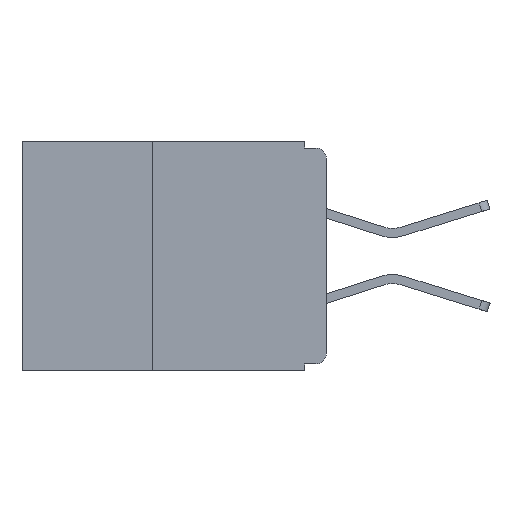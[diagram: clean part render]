
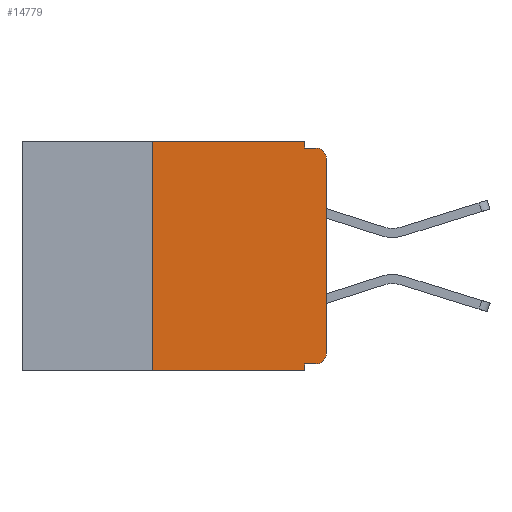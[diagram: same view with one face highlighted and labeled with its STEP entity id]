
A CAD part, left-side view. The second image highlights one B-rep face of the part: STEP entity #14779.
In plain terms, the highlighted planar face has unit normal (-1, 0, 0).
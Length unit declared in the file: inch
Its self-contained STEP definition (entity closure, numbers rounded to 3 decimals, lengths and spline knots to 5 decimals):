
#17 = CARTESIAN_POINT ( 'NONE',  ( 0., 0., -0.32 ) ) ;
#186 = EDGE_CURVE ( 'NONE', #18163, #14115, #7500, .T. ) ;
#317 = CARTESIAN_POINT ( 'NONE',  ( 0., 0.031, -0.01 ) ) ;
#379 = VECTOR ( 'NONE', #11019, 39.37008 ) ;
#574 = LINE ( 'NONE', #5020, #12453 ) ;
#771 = EDGE_CURVE ( 'NONE', #13128, #15462, #13451, .T. ) ;
#1039 = EDGE_CURVE ( 'NONE', #9353, #7749, #12762, .T. ) ;
#1313 = PLANE ( 'NONE',  #11662 ) ;
#2271 = VERTEX_POINT ( 'NONE', #8205 ) ;
#2338 = EDGE_CURVE ( 'NONE', #3840, #9353, #5103, .T. ) ;
#2757 = LINE ( 'NONE', #4085, #10185 ) ;
#2820 = DIRECTION ( 'NONE',  ( 1., 0., 0. ) ) ;
#2853 = LINE ( 'NONE', #16409, #18038 ) ;
#2965 = ORIENTED_EDGE ( 'NONE', *, *, #14677, .F. ) ;
#3108 = CARTESIAN_POINT ( 'NONE',  ( 0., 0.25, -0.33 ) ) ;
#3128 = CIRCLE ( 'NONE', #11853, 0.015 ) ;
#3519 = VECTOR ( 'NONE', #8520, 39.37008 ) ;
#3840 = VERTEX_POINT ( 'NONE', #3108 ) ;
#3855 = CARTESIAN_POINT ( 'NONE',  ( 0., 0.031, -0.33 ) ) ;
#4085 = CARTESIAN_POINT ( 'NONE',  ( 0., 0.031, -0.33 ) ) ;
#4520 = CARTESIAN_POINT ( 'NONE',  ( 0., 0.015, -0.305 ) ) ;
#4841 = LINE ( 'NONE', #17, #379 ) ;
#5020 = CARTESIAN_POINT ( 'NONE',  ( 0., 0.437, -0.33 ) ) ;
#5103 = LINE ( 'NONE', #10503, #9033 ) ;
#5454 = EDGE_LOOP ( 'NONE', ( #10368, #12696, #17447, #10618, #10355, #10684, #18612, #2965, #10865, #7830 ) ) ;
#5501 = EDGE_CURVE ( 'NONE', #12512, #2271, #4841, .T. ) ;
#5509 = CARTESIAN_POINT ( 'NONE',  ( 0., 0.015, -0.025 ) ) ;
#5577 = DIRECTION ( 'NONE',  ( 0., 0., 1. ) ) ;
#6026 = DIRECTION ( 'NONE',  ( 0., 0., -1. ) ) ;
#6424 = CIRCLE ( 'NONE', #17094, 0.015 ) ;
#7005 = DIRECTION ( 'NONE',  ( 0., 0., -1. ) ) ;
#7280 = CARTESIAN_POINT ( 'NONE',  ( 0., 0., 0. ) ) ;
#7500 = LINE ( 'NONE', #7280, #3519 ) ;
#7609 = CARTESIAN_POINT ( 'NONE',  ( 0., 0.25, 0. ) ) ;
#7749 = VERTEX_POINT ( 'NONE', #9363 ) ;
#7830 = ORIENTED_EDGE ( 'NONE', *, *, #10890, .T. ) ;
#8205 = CARTESIAN_POINT ( 'NONE',  ( 0., 0.031, -0.32 ) ) ;
#8284 = CARTESIAN_POINT ( 'NONE',  ( 0., 0.437, 0. ) ) ;
#8520 = DIRECTION ( 'NONE',  ( 0., 0., 1. ) ) ;
#8523 = VERTEX_POINT ( 'NONE', #3855 ) ;
#8824 = FACE_OUTER_BOUND ( 'NONE', #5454, .T. ) ;
#8852 = EDGE_CURVE ( 'NONE', #7749, #13128, #2853, .T. ) ;
#9033 = VECTOR ( 'NONE', #5577, 39.37008 ) ;
#9353 = VERTEX_POINT ( 'NONE', #7609 ) ;
#9363 = CARTESIAN_POINT ( 'NONE',  ( 0., 0.031, 0. ) ) ;
#10142 = CARTESIAN_POINT ( 'NONE',  ( 0., 0.437, 0. ) ) ;
#10185 = VECTOR ( 'NONE', #14400, 39.37008 ) ;
#10355 = ORIENTED_EDGE ( 'NONE', *, *, #1039, .F. ) ;
#10368 = ORIENTED_EDGE ( 'NONE', *, *, #186, .T. ) ;
#10503 = CARTESIAN_POINT ( 'NONE',  ( 0., 0.25, -0.33 ) ) ;
#10618 = ORIENTED_EDGE ( 'NONE', *, *, #8852, .F. ) ;
#10663 = EDGE_CURVE ( 'NONE', #14115, #15462, #6424, .T. ) ;
#10684 = ORIENTED_EDGE ( 'NONE', *, *, #2338, .F. ) ;
#10865 = ORIENTED_EDGE ( 'NONE', *, *, #5501, .F. ) ;
#10890 = EDGE_CURVE ( 'NONE', #12512, #18163, #3128, .T. ) ;
#11019 = DIRECTION ( 'NONE',  ( 0., 1., 0. ) ) ;
#11126 = CARTESIAN_POINT ( 'NONE',  ( 0., 0.015, -0.01 ) ) ;
#11662 = AXIS2_PLACEMENT_3D ( 'NONE', #10142, #2820, #13180 ) ;
#11853 = AXIS2_PLACEMENT_3D ( 'NONE', #4520, #14840, #6026 ) ;
#12453 = VECTOR ( 'NONE', #16789, 39.37008 ) ;
#12512 = VERTEX_POINT ( 'NONE', #16511 ) ;
#12696 = ORIENTED_EDGE ( 'NONE', *, *, #10663, .T. ) ;
#12762 = LINE ( 'NONE', #8284, #16178 ) ;
#13128 = VERTEX_POINT ( 'NONE', #317 ) ;
#13180 = DIRECTION ( 'NONE',  ( 0., 0., -1. ) ) ;
#13451 = LINE ( 'NONE', #16459, #16871 ) ;
#14115 = VERTEX_POINT ( 'NONE', #16015 ) ;
#14400 = DIRECTION ( 'NONE',  ( 0., 0., -1. ) ) ;
#14677 = EDGE_CURVE ( 'NONE', #2271, #8523, #2757, .T. ) ;
#14779 = ADVANCED_FACE ( 'NONE', ( #8824 ), #1313, .F. ) ;
#14840 = DIRECTION ( 'NONE',  ( -1., 0., 0. ) ) ;
#15156 = DIRECTION ( 'NONE',  ( 0., -1., 0. ) ) ;
#15462 = VERTEX_POINT ( 'NONE', #11126 ) ;
#15801 = DIRECTION ( 'NONE',  ( -1., 0., 0. ) ) ;
#16015 = CARTESIAN_POINT ( 'NONE',  ( 0., 0., -0.025 ) ) ;
#16178 = VECTOR ( 'NONE', #15156, 39.37008 ) ;
#16409 = CARTESIAN_POINT ( 'NONE',  ( 0., 0.031, 0. ) ) ;
#16459 = CARTESIAN_POINT ( 'NONE',  ( 0., 0., -0.01 ) ) ;
#16511 = CARTESIAN_POINT ( 'NONE',  ( 0., 0.015, -0.32 ) ) ;
#16572 = DIRECTION ( 'NONE',  ( 0., -1., 0. ) ) ;
#16789 = DIRECTION ( 'NONE',  ( 0., -1., 0. ) ) ;
#16871 = VECTOR ( 'NONE', #16572, 39.37008 ) ;
#17094 = AXIS2_PLACEMENT_3D ( 'NONE', #5509, #15801, #7005 ) ;
#17447 = ORIENTED_EDGE ( 'NONE', *, *, #771, .F. ) ;
#17759 = EDGE_CURVE ( 'NONE', #3840, #8523, #574, .T. ) ;
#17840 = DIRECTION ( 'NONE',  ( 0., 0., -1. ) ) ;
#18038 = VECTOR ( 'NONE', #17840, 39.37008 ) ;
#18163 = VERTEX_POINT ( 'NONE', #18390 ) ;
#18390 = CARTESIAN_POINT ( 'NONE',  ( 0., 0., -0.305 ) ) ;
#18612 = ORIENTED_EDGE ( 'NONE', *, *, #17759, .T. ) ;
